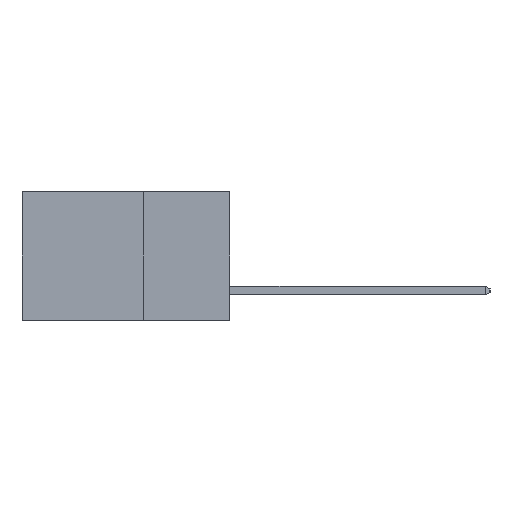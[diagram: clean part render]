
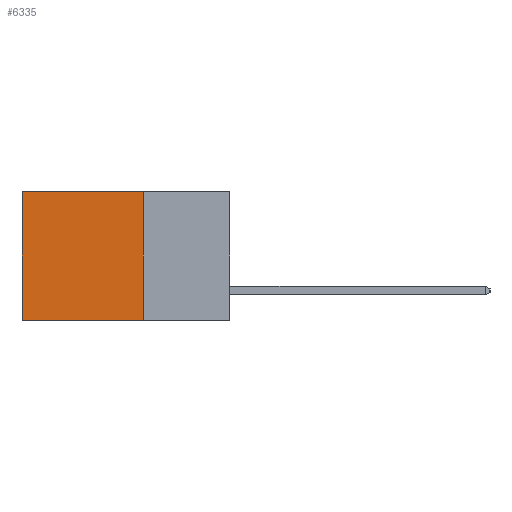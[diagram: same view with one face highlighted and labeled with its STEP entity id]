
A CAD part, left-side view. The second image highlights one B-rep face of the part: STEP entity #6335.
In plain terms, the highlighted planar face has unit normal (-1, 0, 0).
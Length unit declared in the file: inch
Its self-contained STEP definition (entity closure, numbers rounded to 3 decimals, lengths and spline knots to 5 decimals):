
#86 = VECTOR ( 'NONE', #9849, 39.37008 ) ;
#493 = CARTESIAN_POINT ( 'NONE',  ( 0.298, 0.25, 0. ) ) ;
#979 = CARTESIAN_POINT ( 'NONE',  ( 0.298, 0.25, 0. ) ) ;
#1927 = VECTOR ( 'NONE', #4574, 39.37008 ) ;
#1932 = FACE_OUTER_BOUND ( 'NONE', #13853, .T. ) ;
#1969 = DIRECTION ( 'NONE',  ( 0., 1., 0. ) ) ;
#2139 = VERTEX_POINT ( 'NONE', #2371 ) ;
#2371 = CARTESIAN_POINT ( 'NONE',  ( 0.298, 0.6, 0. ) ) ;
#2815 = LINE ( 'NONE', #493, #17304 ) ;
#3100 = CARTESIAN_POINT ( 'NONE',  ( 0.298, 0.6, 0. ) ) ;
#3908 = ORIENTED_EDGE ( 'NONE', *, *, #4473, .F. ) ;
#3976 = LINE ( 'NONE', #6912, #86 ) ;
#4224 = DIRECTION ( 'NONE',  ( 0., 0., -1. ) ) ;
#4473 = EDGE_CURVE ( 'NONE', #7988, #14090, #9316, .T. ) ;
#4574 = DIRECTION ( 'NONE',  ( 0., 0., -1. ) ) ;
#4862 = DIRECTION ( 'NONE',  ( 1., 0., 0. ) ) ;
#5407 = VECTOR ( 'NONE', #16724, 39.37008 ) ;
#6335 = ADVANCED_FACE ( 'NONE', ( #1932 ), #13809, .F. ) ;
#6437 = EDGE_CURVE ( 'NONE', #14090, #11105, #3976, .T. ) ;
#6912 = CARTESIAN_POINT ( 'NONE',  ( 0.298, 0.25, -0.37 ) ) ;
#7166 = EDGE_CURVE ( 'NONE', #7988, #2139, #2815, .T. ) ;
#7988 = VERTEX_POINT ( 'NONE', #18551 ) ;
#9316 = LINE ( 'NONE', #17076, #5407 ) ;
#9723 = LINE ( 'NONE', #3100, #1927 ) ;
#9849 = DIRECTION ( 'NONE',  ( 0., 1., 0. ) ) ;
#11105 = VERTEX_POINT ( 'NONE', #13630 ) ;
#11301 = AXIS2_PLACEMENT_3D ( 'NONE', #979, #4862, #4224 ) ;
#12181 = CARTESIAN_POINT ( 'NONE',  ( 0.298, 0.25, -0.37 ) ) ;
#13178 = ORIENTED_EDGE ( 'NONE', *, *, #13283, .T. ) ;
#13283 = EDGE_CURVE ( 'NONE', #2139, #11105, #9723, .T. ) ;
#13630 = CARTESIAN_POINT ( 'NONE',  ( 0.298, 0.6, -0.37 ) ) ;
#13809 = PLANE ( 'NONE',  #11301 ) ;
#13853 = EDGE_LOOP ( 'NONE', ( #13178, #16170, #3908, #16998 ) ) ;
#14090 = VERTEX_POINT ( 'NONE', #12181 ) ;
#16170 = ORIENTED_EDGE ( 'NONE', *, *, #6437, .F. ) ;
#16724 = DIRECTION ( 'NONE',  ( 0., 0., -1. ) ) ;
#16998 = ORIENTED_EDGE ( 'NONE', *, *, #7166, .T. ) ;
#17076 = CARTESIAN_POINT ( 'NONE',  ( 0.298, 0.25, 0. ) ) ;
#17304 = VECTOR ( 'NONE', #1969, 39.37008 ) ;
#18551 = CARTESIAN_POINT ( 'NONE',  ( 0.298, 0.25, 0. ) ) ;
